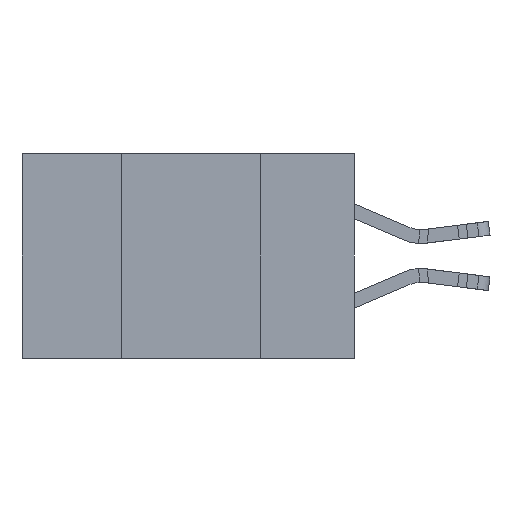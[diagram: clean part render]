
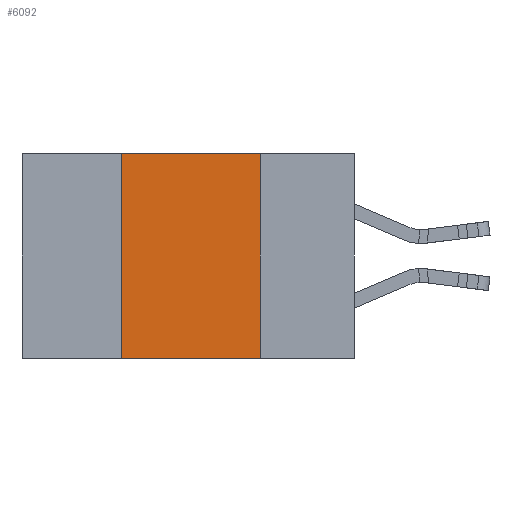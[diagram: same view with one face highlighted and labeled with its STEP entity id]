
A CAD part, left-side view. The second image highlights one B-rep face of the part: STEP entity #6092.
In plain terms, the highlighted planar face has unit normal (-1, 0, 0).
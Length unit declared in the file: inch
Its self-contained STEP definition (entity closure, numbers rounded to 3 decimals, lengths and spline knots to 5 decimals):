
#305 = CARTESIAN_POINT ( 'NONE',  ( 0., 0.6, 0. ) ) ;
#1418 = CARTESIAN_POINT ( 'NONE',  ( 0., 0.6, 0. ) ) ;
#1548 = LINE ( 'NONE', #305, #25767 ) ;
#1562 = ORIENTED_EDGE ( 'NONE', *, *, #11002, .F. ) ;
#4678 = EDGE_CURVE ( 'NONE', #6938, #9482, #22426, .T. ) ;
#5917 = DIRECTION ( 'NONE',  ( 0., -1., 0. ) ) ;
#6092 = ADVANCED_FACE ( 'NONE', ( #8514 ), #27166, .F. ) ;
#6254 = DIRECTION ( 'NONE',  ( 0., 0., -1. ) ) ;
#6938 = VERTEX_POINT ( 'NONE', #13938 ) ;
#7341 = AXIS2_PLACEMENT_3D ( 'NONE', #1418, #20244, #6254 ) ;
#8514 = FACE_OUTER_BOUND ( 'NONE', #27034, .T. ) ;
#8962 = CARTESIAN_POINT ( 'NONE',  ( 0., 0.17, 0. ) ) ;
#9482 = VERTEX_POINT ( 'NONE', #18144 ) ;
#10314 = ORIENTED_EDGE ( 'NONE', *, *, #14170, .F. ) ;
#10806 = VECTOR ( 'NONE', #5917, 39.37008 ) ;
#11002 = EDGE_CURVE ( 'NONE', #6938, #11891, #12761, .T. ) ;
#11891 = VERTEX_POINT ( 'NONE', #19123 ) ;
#12761 = LINE ( 'NONE', #13190, #18197 ) ;
#13190 = CARTESIAN_POINT ( 'NONE',  ( 0., 0.42, 0. ) ) ;
#13733 = LINE ( 'NONE', #23767, #19151 ) ;
#13938 = CARTESIAN_POINT ( 'NONE',  ( 0., 0.42, -0.37 ) ) ;
#14170 = EDGE_CURVE ( 'NONE', #29288, #9482, #13733, .T. ) ;
#14461 = ORIENTED_EDGE ( 'NONE', *, *, #18451, .F. ) ;
#17458 = ORIENTED_EDGE ( 'NONE', *, *, #4678, .T. ) ;
#18144 = CARTESIAN_POINT ( 'NONE',  ( 0., 0.17, -0.37 ) ) ;
#18197 = VECTOR ( 'NONE', #22402, 39.37008 ) ;
#18451 = EDGE_CURVE ( 'NONE', #11891, #29288, #1548, .T. ) ;
#19123 = CARTESIAN_POINT ( 'NONE',  ( 0., 0.42, 0. ) ) ;
#19151 = VECTOR ( 'NONE', #28422, 39.37008 ) ;
#19904 = CARTESIAN_POINT ( 'NONE',  ( 0., 0.6, -0.37 ) ) ;
#20244 = DIRECTION ( 'NONE',  ( 1., 0., 0. ) ) ;
#22402 = DIRECTION ( 'NONE',  ( 0., 0., 1. ) ) ;
#22426 = LINE ( 'NONE', #19904, #10806 ) ;
#23767 = CARTESIAN_POINT ( 'NONE',  ( 0., 0.17, 0. ) ) ;
#23843 = DIRECTION ( 'NONE',  ( 0., -1., 0. ) ) ;
#25767 = VECTOR ( 'NONE', #23843, 39.37008 ) ;
#27034 = EDGE_LOOP ( 'NONE', ( #10314, #14461, #1562, #17458 ) ) ;
#27166 = PLANE ( 'NONE',  #7341 ) ;
#28422 = DIRECTION ( 'NONE',  ( 0., 0., -1. ) ) ;
#29288 = VERTEX_POINT ( 'NONE', #8962 ) ;
